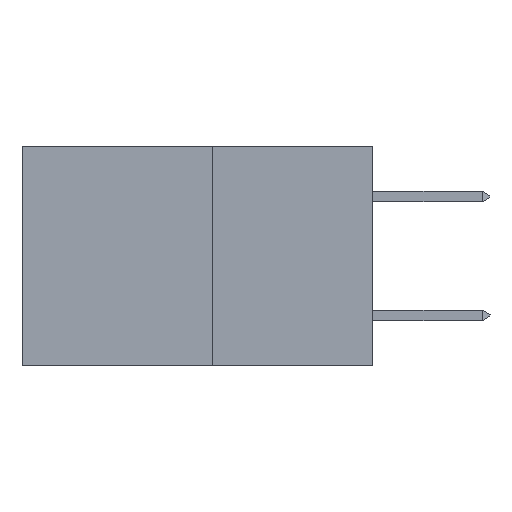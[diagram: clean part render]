
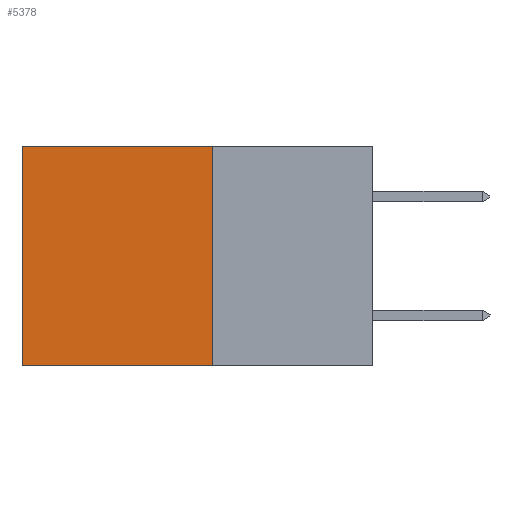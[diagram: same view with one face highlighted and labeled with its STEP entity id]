
A CAD part, left-side view. The second image highlights one B-rep face of the part: STEP entity #5378.
In plain terms, the highlighted planar face has unit normal (-1, 0, 0).
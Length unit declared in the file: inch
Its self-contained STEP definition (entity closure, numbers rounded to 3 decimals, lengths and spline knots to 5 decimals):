
#75 = CARTESIAN_POINT ( 'NONE',  ( 0.277, 0.27, -0.37 ) ) ;
#289 = AXIS2_PLACEMENT_3D ( 'NONE', #7558, #9373, #9338 ) ;
#600 = CARTESIAN_POINT ( 'NONE',  ( 0.277, 0.27, 0. ) ) ;
#671 = DIRECTION ( 'NONE',  ( 0., 1., 0. ) ) ;
#962 = CARTESIAN_POINT ( 'NONE',  ( 0.277, 0.27, -0.37 ) ) ;
#1295 = ORIENTED_EDGE ( 'NONE', *, *, #14011, .F. ) ;
#1446 = DIRECTION ( 'NONE',  ( 0., 0., -1. ) ) ;
#1557 = CARTESIAN_POINT ( 'NONE',  ( 0.277, 0.27, -0.37 ) ) ;
#2634 = DIRECTION ( 'NONE',  ( 0., 1., 0. ) ) ;
#3181 = VERTEX_POINT ( 'NONE', #15773 ) ;
#3228 = VECTOR ( 'NONE', #2634, 39.37008 ) ;
#3739 = LINE ( 'NONE', #962, #3228 ) ;
#5378 = ADVANCED_FACE ( 'NONE', ( #8182 ), #9401, .F. ) ;
#6077 = EDGE_CURVE ( 'NONE', #17265, #18625, #12850, .T. ) ;
#7310 = EDGE_CURVE ( 'NONE', #14657, #3181, #19239, .T. ) ;
#7558 = CARTESIAN_POINT ( 'NONE',  ( 0.277, 0.27, -0.37 ) ) ;
#7708 = LINE ( 'NONE', #600, #17094 ) ;
#7836 = ORIENTED_EDGE ( 'NONE', *, *, #12650, .T. ) ;
#8164 = CARTESIAN_POINT ( 'NONE',  ( 0.277, 0.27, 0. ) ) ;
#8182 = FACE_OUTER_BOUND ( 'NONE', #8503, .T. ) ;
#8503 = EDGE_LOOP ( 'NONE', ( #9339, #1295, #19970, #7836 ) ) ;
#9338 = DIRECTION ( 'NONE',  ( 0., 0., -1. ) ) ;
#9339 = ORIENTED_EDGE ( 'NONE', *, *, #7310, .T. ) ;
#9373 = DIRECTION ( 'NONE',  ( 1., 0., 0. ) ) ;
#9401 = PLANE ( 'NONE',  #289 ) ;
#12421 = DIRECTION ( 'NONE',  ( 0., 0., -1. ) ) ;
#12650 = EDGE_CURVE ( 'NONE', #17265, #14657, #7708, .T. ) ;
#12850 = LINE ( 'NONE', #75, #13390 ) ;
#12938 = CARTESIAN_POINT ( 'NONE',  ( 0.277, 0.59, -0.37 ) ) ;
#13390 = VECTOR ( 'NONE', #1446, 39.37008 ) ;
#14011 = EDGE_CURVE ( 'NONE', #18625, #3181, #3739, .T. ) ;
#14657 = VERTEX_POINT ( 'NONE', #17375 ) ;
#14904 = VECTOR ( 'NONE', #12421, 39.37008 ) ;
#15773 = CARTESIAN_POINT ( 'NONE',  ( 0.277, 0.59, -0.37 ) ) ;
#17094 = VECTOR ( 'NONE', #671, 39.37008 ) ;
#17265 = VERTEX_POINT ( 'NONE', #8164 ) ;
#17375 = CARTESIAN_POINT ( 'NONE',  ( 0.277, 0.59, 0. ) ) ;
#18625 = VERTEX_POINT ( 'NONE', #1557 ) ;
#19239 = LINE ( 'NONE', #12938, #14904 ) ;
#19970 = ORIENTED_EDGE ( 'NONE', *, *, #6077, .F. ) ;
